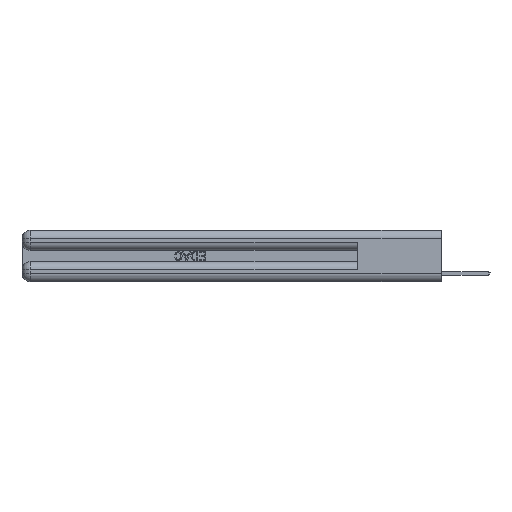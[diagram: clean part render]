
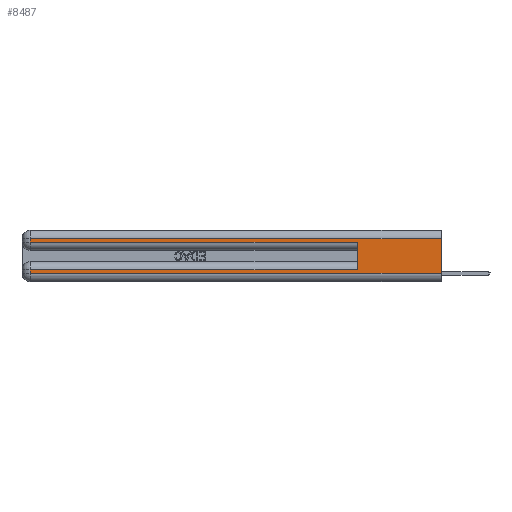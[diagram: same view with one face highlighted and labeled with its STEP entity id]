
A CAD part, left-side view. The second image highlights one B-rep face of the part: STEP entity #8487.
In plain terms, the highlighted planar face has unit normal (-1, 0, 0).
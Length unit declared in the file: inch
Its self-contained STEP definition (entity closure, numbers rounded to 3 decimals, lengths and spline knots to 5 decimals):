
#423 = ORIENTED_EDGE ( 'NONE', *, *, #10208, .T. ) ;
#780 = DIRECTION ( 'NONE',  ( 0., 0., 1. ) ) ;
#1691 = LINE ( 'NONE', #31722, #26585 ) ;
#2374 = CARTESIAN_POINT ( 'NONE',  ( 0., 0., 0.31 ) ) ;
#2630 = CARTESIAN_POINT ( 'NONE',  ( 0., 0., 0.37 ) ) ;
#3359 = CARTESIAN_POINT ( 'NONE',  ( 0., 2.94, 0.31 ) ) ;
#4234 = VECTOR ( 'NONE', #5108, 39.37008 ) ;
#5108 = DIRECTION ( 'NONE',  ( 0., 0., -1. ) ) ;
#5445 = CARTESIAN_POINT ( 'NONE',  ( 0., 0., 0.37 ) ) ;
#5551 = VERTEX_POINT ( 'NONE', #20878 ) ;
#5593 = CARTESIAN_POINT ( 'NONE',  ( 0., 2.94, 0.06 ) ) ;
#5628 = EDGE_CURVE ( 'NONE', #6950, #31762, #6163, .T. ) ;
#6163 = LINE ( 'NONE', #25973, #8863 ) ;
#6209 = VERTEX_POINT ( 'NONE', #2374 ) ;
#6508 = CARTESIAN_POINT ( 'NONE',  ( 0., 2.94, 0.285 ) ) ;
#6950 = VERTEX_POINT ( 'NONE', #6508 ) ;
#6972 = VERTEX_POINT ( 'NONE', #13763 ) ;
#7373 = ORIENTED_EDGE ( 'NONE', *, *, #26478, .T. ) ;
#7604 = DIRECTION ( 'NONE',  ( 0., 0., -1. ) ) ;
#7932 = DIRECTION ( 'NONE',  ( 1., 0., 0. ) ) ;
#8075 = ORIENTED_EDGE ( 'NONE', *, *, #12564, .T. ) ;
#8267 = CARTESIAN_POINT ( 'NONE',  ( 0., 0.6, 0.285 ) ) ;
#8487 = ADVANCED_FACE ( 'NONE', ( #24875 ), #20107, .F. ) ;
#8863 = VECTOR ( 'NONE', #15354, 39.37008 ) ;
#9117 = EDGE_CURVE ( 'NONE', #5551, #31762, #25611, .T. ) ;
#9615 = ORIENTED_EDGE ( 'NONE', *, *, #29098, .T. ) ;
#10208 = EDGE_CURVE ( 'NONE', #5551, #6972, #11407, .T. ) ;
#10567 = CARTESIAN_POINT ( 'NONE',  ( 0., 0., 0.31 ) ) ;
#10923 = AXIS2_PLACEMENT_3D ( 'NONE', #5445, #7932, #7604 ) ;
#11407 = LINE ( 'NONE', #31724, #28254 ) ;
#11496 = VECTOR ( 'NONE', #780, 39.37008 ) ;
#12075 = CARTESIAN_POINT ( 'NONE',  ( 0., 0., 0.06 ) ) ;
#12563 = EDGE_CURVE ( 'NONE', #21899, #12756, #25430, .T. ) ;
#12564 = EDGE_CURVE ( 'NONE', #23166, #6950, #1691, .T. ) ;
#12756 = VERTEX_POINT ( 'NONE', #17744 ) ;
#13394 = LINE ( 'NONE', #17123, #4234 ) ;
#13763 = CARTESIAN_POINT ( 'NONE',  ( 0., 2.94, 0.085 ) ) ;
#14295 = VECTOR ( 'NONE', #27038, 39.37008 ) ;
#14310 = VECTOR ( 'NONE', #19879, 39.37008 ) ;
#15354 = DIRECTION ( 'NONE',  ( 0., -1., 0. ) ) ;
#17123 = CARTESIAN_POINT ( 'NONE',  ( 0., 2.94, 0.37 ) ) ;
#17744 = CARTESIAN_POINT ( 'NONE',  ( 0., 0., 0.06 ) ) ;
#19879 = DIRECTION ( 'NONE',  ( 0., 1., 0. ) ) ;
#20097 = CARTESIAN_POINT ( 'NONE',  ( 0., 0.6, 0.145 ) ) ;
#20107 = PLANE ( 'NONE',  #10923 ) ;
#20878 = CARTESIAN_POINT ( 'NONE',  ( 0., 0.6, 0.085 ) ) ;
#21741 = EDGE_LOOP ( 'NONE', ( #21904, #9615, #8075, #25154, #25672, #423, #7373, #24234 ) ) ;
#21899 = VERTEX_POINT ( 'NONE', #5593 ) ;
#21904 = ORIENTED_EDGE ( 'NONE', *, *, #25775, .F. ) ;
#22097 = DIRECTION ( 'NONE',  ( 0., 0., -1. ) ) ;
#22258 = DIRECTION ( 'NONE',  ( 0., 0., -1. ) ) ;
#22378 = LINE ( 'NONE', #10567, #14310 ) ;
#23166 = VERTEX_POINT ( 'NONE', #3359 ) ;
#24234 = ORIENTED_EDGE ( 'NONE', *, *, #12563, .T. ) ;
#24875 = FACE_OUTER_BOUND ( 'NONE', #21741, .T. ) ;
#25154 = ORIENTED_EDGE ( 'NONE', *, *, #5628, .T. ) ;
#25319 = LINE ( 'NONE', #2630, #31100 ) ;
#25430 = LINE ( 'NONE', #12075, #14295 ) ;
#25611 = LINE ( 'NONE', #20097, #11496 ) ;
#25672 = ORIENTED_EDGE ( 'NONE', *, *, #9117, .F. ) ;
#25775 = EDGE_CURVE ( 'NONE', #6209, #12756, #25319, .T. ) ;
#25973 = CARTESIAN_POINT ( 'NONE',  ( 0., 0., 0.285 ) ) ;
#26478 = EDGE_CURVE ( 'NONE', #6972, #21899, #13394, .T. ) ;
#26585 = VECTOR ( 'NONE', #22097, 39.37008 ) ;
#27038 = DIRECTION ( 'NONE',  ( 0., -1., 0. ) ) ;
#28254 = VECTOR ( 'NONE', #29715, 39.37008 ) ;
#29098 = EDGE_CURVE ( 'NONE', #6209, #23166, #22378, .T. ) ;
#29715 = DIRECTION ( 'NONE',  ( 0., 1., 0. ) ) ;
#31100 = VECTOR ( 'NONE', #22258, 39.37008 ) ;
#31722 = CARTESIAN_POINT ( 'NONE',  ( 0., 2.94, 0.37 ) ) ;
#31724 = CARTESIAN_POINT ( 'NONE',  ( 0., 0., 0.085 ) ) ;
#31762 = VERTEX_POINT ( 'NONE', #8267 ) ;
